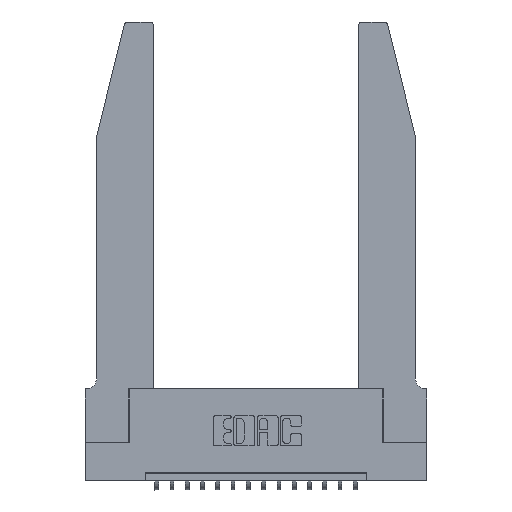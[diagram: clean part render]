
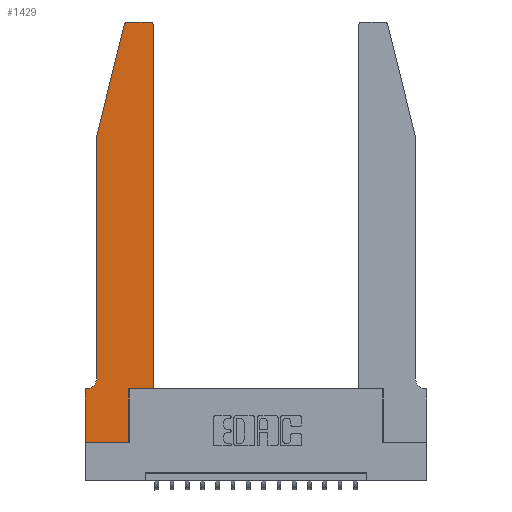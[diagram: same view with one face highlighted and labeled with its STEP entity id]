
A CAD part, top view. The second image highlights one B-rep face of the part: STEP entity #1429.
In plain terms, the highlighted planar face has unit normal (0, 0, 1).
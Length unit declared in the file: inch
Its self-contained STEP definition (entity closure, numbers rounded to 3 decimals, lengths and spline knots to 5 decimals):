
#290 = ORIENTED_EDGE ( 'NONE', *, *, #947, .T. ) ;
#381 = CARTESIAN_POINT ( 'NONE',  ( 0.4505, 2.72, 0.37 ) ) ;
#464 = AXIS2_PLACEMENT_3D ( 'NONE', #14585, #8718, #10144 ) ;
#569 = DIRECTION ( 'NONE',  ( 0., 0., 1. ) ) ;
#575 = CARTESIAN_POINT ( 'NONE',  ( 0., 0., 0.37 ) ) ;
#715 = DIRECTION ( 'NONE',  ( 0., 0., -1. ) ) ;
#733 = CARTESIAN_POINT ( 'NONE',  ( 0.284, 2.72, 0.37 ) ) ;
#844 = EDGE_CURVE ( 'NONE', #9264, #10544, #7103, .T. ) ;
#947 = EDGE_CURVE ( 'NONE', #14576, #13072, #12448, .T. ) ;
#1001 = ORIENTED_EDGE ( 'NONE', *, *, #13602, .T. ) ;
#1346 = VECTOR ( 'NONE', #3991, 39.37008 ) ;
#1429 = ADVANCED_FACE ( 'NONE', ( #17029 ), #6557, .T. ) ;
#1465 = EDGE_CURVE ( 'NONE', #4742, #6917, #6859, .T. ) ;
#1737 = CARTESIAN_POINT ( 'NONE',  ( 0.0755, 0.42, 0.37 ) ) ;
#2220 = DIRECTION ( 'NONE',  ( 1., 0., 0. ) ) ;
#2391 = DIRECTION ( 'NONE',  ( 1., 0., 0. ) ) ;
#2590 = LINE ( 'NONE', #12638, #10196 ) ;
#2692 = DIRECTION ( 'NONE',  ( 0., -1., 0. ) ) ;
#2755 = ORIENTED_EDGE ( 'NONE', *, *, #11110, .T. ) ;
#3235 = VERTEX_POINT ( 'NONE', #1737 ) ;
#3288 = LINE ( 'NONE', #7178, #13924 ) ;
#3405 = DIRECTION ( 'NONE',  ( 1., 0., 0. ) ) ;
#3620 = DIRECTION ( 'NONE',  ( -1., 0., 0. ) ) ;
#3991 = DIRECTION ( 'NONE',  ( -1., 0., 0. ) ) ;
#4228 = DIRECTION ( 'NONE',  ( 0., 1., 0. ) ) ;
#4566 = VECTOR ( 'NONE', #4684, 39.37008 ) ;
#4684 = DIRECTION ( 'NONE',  ( 0., 1., 0. ) ) ;
#4742 = VERTEX_POINT ( 'NONE', #575 ) ;
#5142 = DIRECTION ( 'NONE',  ( -1., 0., 0. ) ) ;
#5245 = CARTESIAN_POINT ( 'NONE',  ( 0.284, 2.75, 0.37 ) ) ;
#5252 = VERTEX_POINT ( 'NONE', #381 ) ;
#5297 = ORIENTED_EDGE ( 'NONE', *, *, #9566, .T. ) ;
#5471 = VECTOR ( 'NONE', #9669, 39.37008 ) ;
#5521 = CARTESIAN_POINT ( 'NONE',  ( 0.2865, 0.35, 0.37 ) ) ;
#5815 = DIRECTION ( 'NONE',  ( -0.239, -0.971, 0. ) ) ;
#6157 = VERTEX_POINT ( 'NONE', #9835 ) ;
#6350 = VERTEX_POINT ( 'NONE', #12885 ) ;
#6557 = PLANE ( 'NONE',  #11710 ) ;
#6852 = VECTOR ( 'NONE', #2692, 39.37008 ) ;
#6859 = LINE ( 'NONE', #8553, #5471 ) ;
#6917 = VERTEX_POINT ( 'NONE', #14194 ) ;
#6994 = VERTEX_POINT ( 'NONE', #5521 ) ;
#7103 = LINE ( 'NONE', #17026, #8731 ) ;
#7178 = CARTESIAN_POINT ( 'NONE',  ( 0.0755, 2., 0.37 ) ) ;
#7916 = CIRCLE ( 'NONE', #17043, 0.07 ) ;
#8162 = VECTOR ( 'NONE', #2391, 39.37008 ) ;
#8223 = CARTESIAN_POINT ( 'NONE',  ( 0.4205, 2.75, 0.37 ) ) ;
#8423 = ORIENTED_EDGE ( 'NONE', *, *, #10117, .T. ) ;
#8450 = CARTESIAN_POINT ( 'NONE',  ( 0.2605, 2.75, 0.37 ) ) ;
#8553 = CARTESIAN_POINT ( 'NONE',  ( 0., 0., 0.37 ) ) ;
#8718 = DIRECTION ( 'NONE',  ( 0., 0., 1. ) ) ;
#8723 = LINE ( 'NONE', #17669, #6852 ) ;
#8731 = VECTOR ( 'NONE', #5142, 39.37008 ) ;
#8779 = EDGE_CURVE ( 'NONE', #5252, #14576, #15104, .T. ) ;
#9070 = ORIENTED_EDGE ( 'NONE', *, *, #1465, .T. ) ;
#9078 = CARTESIAN_POINT ( 'NONE',  ( 0.2865, 0.35, 0.37 ) ) ;
#9264 = VERTEX_POINT ( 'NONE', #16476 ) ;
#9566 = EDGE_CURVE ( 'NONE', #6350, #5252, #14184, .T. ) ;
#9669 = DIRECTION ( 'NONE',  ( 1., 0., 0. ) ) ;
#9686 = ORIENTED_EDGE ( 'NONE', *, *, #8779, .T. ) ;
#9835 = CARTESIAN_POINT ( 'NONE',  ( 0.25487, 2.72718, 0.37 ) ) ;
#10117 = EDGE_CURVE ( 'NONE', #6994, #6350, #18067, .T. ) ;
#10144 = DIRECTION ( 'NONE',  ( 1., 0., 0. ) ) ;
#10196 = VECTOR ( 'NONE', #17141, 39.37008 ) ;
#10410 = EDGE_CURVE ( 'NONE', #3235, #9264, #7916, .T. ) ;
#10544 = VERTEX_POINT ( 'NONE', #12581 ) ;
#10802 = CARTESIAN_POINT ( 'NONE',  ( 0.0755, 2., 0.37 ) ) ;
#11051 = DIRECTION ( 'NONE',  ( 0., 0., 1. ) ) ;
#11110 = EDGE_CURVE ( 'NONE', #6157, #17766, #3288, .T. ) ;
#11592 = ORIENTED_EDGE ( 'NONE', *, *, #15023, .T. ) ;
#11710 = AXIS2_PLACEMENT_3D ( 'NONE', #12233, #569, #3405 ) ;
#11754 = CIRCLE ( 'NONE', #17957, 0.03 ) ;
#12233 = CARTESIAN_POINT ( 'NONE',  ( 0., 0.35, 0.37 ) ) ;
#12318 = ORIENTED_EDGE ( 'NONE', *, *, #18797, .T. ) ;
#12337 = VECTOR ( 'NONE', #4228, 39.37008 ) ;
#12448 = LINE ( 'NONE', #8450, #1346 ) ;
#12526 = ORIENTED_EDGE ( 'NONE', *, *, #844, .T. ) ;
#12581 = CARTESIAN_POINT ( 'NONE',  ( 0., 0.35, 0.37 ) ) ;
#12638 = CARTESIAN_POINT ( 'NONE',  ( 0., 0., 0.37 ) ) ;
#12827 = CARTESIAN_POINT ( 'NONE',  ( 0.4505, 0.35, 0.37 ) ) ;
#12885 = CARTESIAN_POINT ( 'NONE',  ( 0.4505, 0.35, 0.37 ) ) ;
#12899 = LINE ( 'NONE', #9078, #4566 ) ;
#13072 = VERTEX_POINT ( 'NONE', #5245 ) ;
#13404 = ORIENTED_EDGE ( 'NONE', *, *, #10410, .T. ) ;
#13602 = EDGE_CURVE ( 'NONE', #6917, #6994, #12899, .T. ) ;
#13891 = CARTESIAN_POINT ( 'NONE',  ( 0.0055, 0.42, 0.37 ) ) ;
#13924 = VECTOR ( 'NONE', #5815, 39.37008 ) ;
#14184 = LINE ( 'NONE', #12827, #12337 ) ;
#14194 = CARTESIAN_POINT ( 'NONE',  ( 0.2865, 0., 0.37 ) ) ;
#14490 = EDGE_CURVE ( 'NONE', #13072, #6157, #11754, .T. ) ;
#14576 = VERTEX_POINT ( 'NONE', #8223 ) ;
#14585 = CARTESIAN_POINT ( 'NONE',  ( 0.4205, 2.72, 0.37 ) ) ;
#15023 = EDGE_CURVE ( 'NONE', #17766, #3235, #8723, .T. ) ;
#15104 = CIRCLE ( 'NONE', #464, 0.03 ) ;
#15186 = EDGE_LOOP ( 'NONE', ( #290, #15286, #2755, #11592, #13404, #12526, #12318, #9070, #1001, #8423, #5297, #9686 ) ) ;
#15286 = ORIENTED_EDGE ( 'NONE', *, *, #14490, .T. ) ;
#16476 = CARTESIAN_POINT ( 'NONE',  ( 0.0055, 0.35, 0.37 ) ) ;
#17026 = CARTESIAN_POINT ( 'NONE',  ( 0.0755, 0.35, 0.37 ) ) ;
#17029 = FACE_OUTER_BOUND ( 'NONE', #15186, .T. ) ;
#17043 = AXIS2_PLACEMENT_3D ( 'NONE', #13891, #715, #3620 ) ;
#17141 = DIRECTION ( 'NONE',  ( 0., -1., 0. ) ) ;
#17669 = CARTESIAN_POINT ( 'NONE',  ( 0.0755, 2., 0.37 ) ) ;
#17766 = VERTEX_POINT ( 'NONE', #10802 ) ;
#17957 = AXIS2_PLACEMENT_3D ( 'NONE', #733, #11051, #2220 ) ;
#18067 = LINE ( 'NONE', #18658, #8162 ) ;
#18658 = CARTESIAN_POINT ( 'NONE',  ( 0.4505, 0.35, 0.37 ) ) ;
#18797 = EDGE_CURVE ( 'NONE', #10544, #4742, #2590, .T. ) ;
